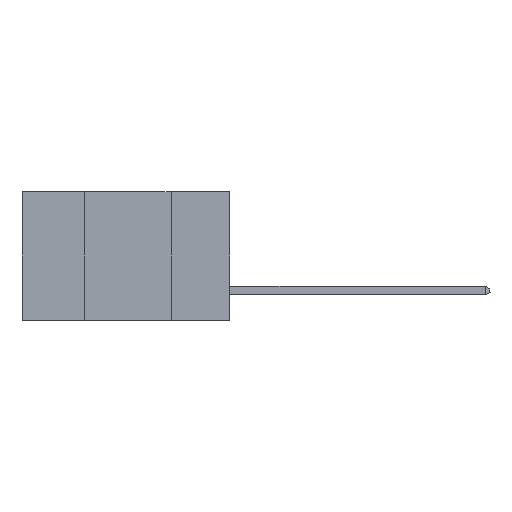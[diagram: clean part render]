
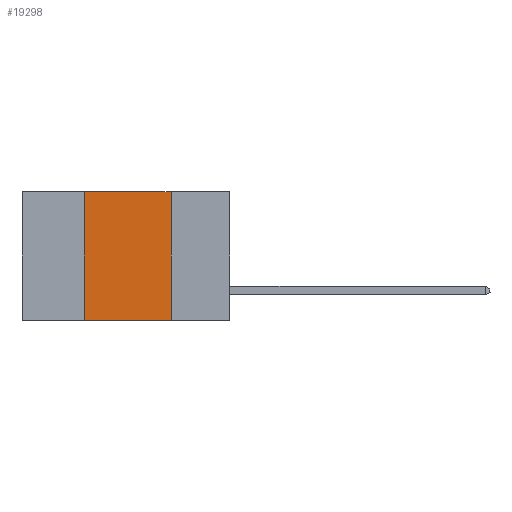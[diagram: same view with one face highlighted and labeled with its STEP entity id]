
A CAD part, left-side view. The second image highlights one B-rep face of the part: STEP entity #19298.
In plain terms, the highlighted planar face has unit normal (-1, 0, 0).
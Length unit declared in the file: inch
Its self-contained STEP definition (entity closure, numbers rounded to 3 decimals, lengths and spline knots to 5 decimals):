
#322 = EDGE_CURVE ( 'NONE', #11289, #6946, #20657, .T. ) ;
#1193 = FACE_OUTER_BOUND ( 'NONE', #6700, .T. ) ;
#1223 = ORIENTED_EDGE ( 'NONE', *, *, #9718, .T. ) ;
#1878 = CARTESIAN_POINT ( 'NONE',  ( 0., 0.17, 0. ) ) ;
#2124 = ORIENTED_EDGE ( 'NONE', *, *, #322, .F. ) ;
#4631 = EDGE_CURVE ( 'NONE', #14356, #4743, #18615, .T. ) ;
#4743 = VERTEX_POINT ( 'NONE', #11148 ) ;
#5415 = LINE ( 'NONE', #13719, #20314 ) ;
#6700 = EDGE_LOOP ( 'NONE', ( #10842, #19643, #2124, #1223 ) ) ;
#6946 = VERTEX_POINT ( 'NONE', #8470 ) ;
#7153 = DIRECTION ( 'NONE',  ( 0., 0., -1. ) ) ;
#7361 = PLANE ( 'NONE',  #10806 ) ;
#7835 = CARTESIAN_POINT ( 'NONE',  ( 0., 0.42, 0. ) ) ;
#8470 = CARTESIAN_POINT ( 'NONE',  ( 0., 0.42, 0. ) ) ;
#8831 = DIRECTION ( 'NONE',  ( 0., -1., 0. ) ) ;
#9718 = EDGE_CURVE ( 'NONE', #11289, #4743, #5415, .T. ) ;
#9764 = CARTESIAN_POINT ( 'NONE',  ( 0., 0.17, 0. ) ) ;
#10660 = DIRECTION ( 'NONE',  ( 0., -1., 0. ) ) ;
#10806 = AXIS2_PLACEMENT_3D ( 'NONE', #18920, #20570, #7153 ) ;
#10842 = ORIENTED_EDGE ( 'NONE', *, *, #4631, .F. ) ;
#11028 = CARTESIAN_POINT ( 'NONE',  ( 0., 0.42, -0.37 ) ) ;
#11148 = CARTESIAN_POINT ( 'NONE',  ( 0., 0.17, -0.37 ) ) ;
#11289 = VERTEX_POINT ( 'NONE', #11028 ) ;
#11435 = VECTOR ( 'NONE', #19536, 39.37008 ) ;
#12869 = VECTOR ( 'NONE', #10660, 39.37008 ) ;
#13719 = CARTESIAN_POINT ( 'NONE',  ( 0., 0.6, -0.37 ) ) ;
#14356 = VERTEX_POINT ( 'NONE', #9764 ) ;
#15023 = DIRECTION ( 'NONE',  ( 0., 0., -1. ) ) ;
#15281 = VECTOR ( 'NONE', #15023, 39.37008 ) ;
#16959 = EDGE_CURVE ( 'NONE', #6946, #14356, #19005, .T. ) ;
#18615 = LINE ( 'NONE', #1878, #15281 ) ;
#18684 = CARTESIAN_POINT ( 'NONE',  ( 0., 0.6, 0. ) ) ;
#18920 = CARTESIAN_POINT ( 'NONE',  ( 0., 0.6, 0. ) ) ;
#19005 = LINE ( 'NONE', #18684, #12869 ) ;
#19298 = ADVANCED_FACE ( 'NONE', ( #1193 ), #7361, .F. ) ;
#19536 = DIRECTION ( 'NONE',  ( 0., 0., 1. ) ) ;
#19643 = ORIENTED_EDGE ( 'NONE', *, *, #16959, .F. ) ;
#20314 = VECTOR ( 'NONE', #8831, 39.37008 ) ;
#20570 = DIRECTION ( 'NONE',  ( 1., 0., 0. ) ) ;
#20657 = LINE ( 'NONE', #7835, #11435 ) ;
